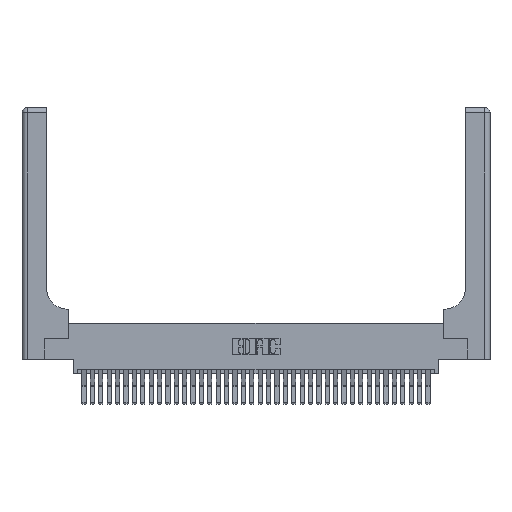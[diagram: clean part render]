
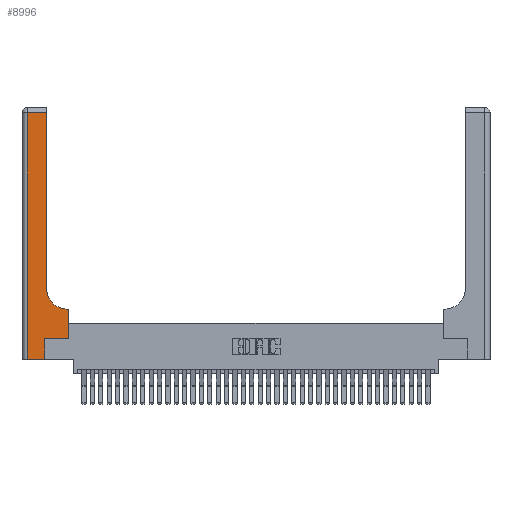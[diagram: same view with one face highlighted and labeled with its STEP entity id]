
A CAD part, top view. The second image highlights one B-rep face of the part: STEP entity #8996.
In plain terms, the highlighted planar face has unit normal (0, 0, 1).
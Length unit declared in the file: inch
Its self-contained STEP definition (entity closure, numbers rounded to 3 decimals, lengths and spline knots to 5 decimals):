
#101 = LINE ( 'NONE', #31288, #15842 ) ;
#147 = LINE ( 'NONE', #14560, #558 ) ;
#292 = DIRECTION ( 'NONE',  ( -1., 0., 0. ) ) ;
#504 = ORIENTED_EDGE ( 'NONE', *, *, #34181, .T. ) ;
#558 = VECTOR ( 'NONE', #29402, 39.37008 ) ;
#624 = PLANE ( 'NONE',  #20999 ) ;
#1263 = DIRECTION ( 'NONE',  ( 1., 0., 0. ) ) ;
#1384 = EDGE_CURVE ( 'NONE', #15365, #7239, #147, .T. ) ;
#1954 = DIRECTION ( 'NONE',  ( 0., 0., -1. ) ) ;
#2042 = ORIENTED_EDGE ( 'NONE', *, *, #28982, .T. ) ;
#2110 = VERTEX_POINT ( 'NONE', #31907 ) ;
#2612 = DIRECTION ( 'NONE',  ( 0., 1., 0. ) ) ;
#3380 = ORIENTED_EDGE ( 'NONE', *, *, #1384, .T. ) ;
#4541 = CARTESIAN_POINT ( 'NONE',  ( 0.5585, 0.6, 0.37 ) ) ;
#6679 = DIRECTION ( 'NONE',  ( -1., 0., 0. ) ) ;
#7239 = VERTEX_POINT ( 'NONE', #7266 ) ;
#7266 = CARTESIAN_POINT ( 'NONE',  ( 0.269, 0., 0.37 ) ) ;
#7744 = CARTESIAN_POINT ( 'NONE',  ( 0., 3., 0.37 ) ) ;
#7892 = CARTESIAN_POINT ( 'NONE',  ( 0.2915, 0.6, 0.37 ) ) ;
#8210 = DIRECTION ( 'NONE',  ( -1., 0., 0. ) ) ;
#8481 = EDGE_CURVE ( 'NONE', #35410, #12416, #36469, .T. ) ;
#8996 = ADVANCED_FACE ( 'NONE', ( #12346 ), #624, .F. ) ;
#9677 = CIRCLE ( 'NONE', #15963, 0.25 ) ;
#10254 = VECTOR ( 'NONE', #22843, 39.37008 ) ;
#10295 = CARTESIAN_POINT ( 'NONE',  ( 0.269, 0.25, 0.37 ) ) ;
#10533 = DIRECTION ( 'NONE',  ( 0., 1., 0. ) ) ;
#11462 = VECTOR ( 'NONE', #10533, 39.37008 ) ;
#12210 = CARTESIAN_POINT ( 'NONE',  ( 0.5415, 0.85, 0.37 ) ) ;
#12346 = FACE_OUTER_BOUND ( 'NONE', #29257, .T. ) ;
#12416 = VERTEX_POINT ( 'NONE', #35075 ) ;
#12736 = VECTOR ( 'NONE', #2612, 39.37008 ) ;
#12944 = ORIENTED_EDGE ( 'NONE', *, *, #18998, .T. ) ;
#13039 = VECTOR ( 'NONE', #21539, 39.37008 ) ;
#14560 = CARTESIAN_POINT ( 'NONE',  ( 0., 0., 0.37 ) ) ;
#15365 = VERTEX_POINT ( 'NONE', #15986 ) ;
#15382 = CARTESIAN_POINT ( 'NONE',  ( 0.269, 0.25, 0.37 ) ) ;
#15471 = ORIENTED_EDGE ( 'NONE', *, *, #28956, .T. ) ;
#15842 = VECTOR ( 'NONE', #16660, 39.37008 ) ;
#15963 = AXIS2_PLACEMENT_3D ( 'NONE', #12210, #32925, #1263 ) ;
#15986 = CARTESIAN_POINT ( 'NONE',  ( 0.06, 0., 0.37 ) ) ;
#16660 = DIRECTION ( 'NONE',  ( 0., -1., 0. ) ) ;
#16808 = LINE ( 'NONE', #7892, #33022 ) ;
#18998 = EDGE_CURVE ( 'NONE', #30718, #38318, #32044, .T. ) ;
#19745 = CARTESIAN_POINT ( 'NONE',  ( 0.269, 0., 0.37 ) ) ;
#20999 = AXIS2_PLACEMENT_3D ( 'NONE', #7744, #1954, #6679 ) ;
#21539 = DIRECTION ( 'NONE',  ( 1., 0., 0. ) ) ;
#22843 = DIRECTION ( 'NONE',  ( 0., 1., 0. ) ) ;
#23670 = VECTOR ( 'NONE', #8210, 39.37008 ) ;
#23707 = LINE ( 'NONE', #19745, #10254 ) ;
#23915 = CARTESIAN_POINT ( 'NONE',  ( 0.2915, 0.85, 0.37 ) ) ;
#24490 = VERTEX_POINT ( 'NONE', #25920 ) ;
#24520 = EDGE_CURVE ( 'NONE', #35234, #24490, #16808, .T. ) ;
#25920 = CARTESIAN_POINT ( 'NONE',  ( 0.5415, 0.6, 0.37 ) ) ;
#26188 = CARTESIAN_POINT ( 'NONE',  ( 0.5585, 0.25, 0.37 ) ) ;
#28956 = EDGE_CURVE ( 'NONE', #7239, #30718, #23707, .T. ) ;
#28982 = EDGE_CURVE ( 'NONE', #2110, #15365, #101, .T. ) ;
#29152 = EDGE_CURVE ( 'NONE', #12416, #2110, #31587, .T. ) ;
#29257 = EDGE_LOOP ( 'NONE', ( #30025, #30339, #2042, #3380, #15471, #12944, #504, #30151, #35249 ) ) ;
#29402 = DIRECTION ( 'NONE',  ( 1., 0., 0. ) ) ;
#30008 = EDGE_CURVE ( 'NONE', #24490, #35410, #9677, .T. ) ;
#30025 = ORIENTED_EDGE ( 'NONE', *, *, #8481, .T. ) ;
#30151 = ORIENTED_EDGE ( 'NONE', *, *, #24520, .T. ) ;
#30339 = ORIENTED_EDGE ( 'NONE', *, *, #29152, .T. ) ;
#30718 = VERTEX_POINT ( 'NONE', #10295 ) ;
#31288 = CARTESIAN_POINT ( 'NONE',  ( 0.06, 3., 0.37 ) ) ;
#31587 = LINE ( 'NONE', #37923, #23670 ) ;
#31907 = CARTESIAN_POINT ( 'NONE',  ( 0.06, 2.94, 0.37 ) ) ;
#32044 = LINE ( 'NONE', #15382, #13039 ) ;
#32925 = DIRECTION ( 'NONE',  ( 0., 0., -1. ) ) ;
#33022 = VECTOR ( 'NONE', #292, 39.37008 ) ;
#33115 = LINE ( 'NONE', #26188, #12736 ) ;
#34181 = EDGE_CURVE ( 'NONE', #38318, #35234, #33115, .T. ) ;
#34693 = CARTESIAN_POINT ( 'NONE',  ( 0.2915, 3., 0.37 ) ) ;
#35075 = CARTESIAN_POINT ( 'NONE',  ( 0.2915, 2.94, 0.37 ) ) ;
#35137 = CARTESIAN_POINT ( 'NONE',  ( 0.5585, 0.25, 0.37 ) ) ;
#35234 = VERTEX_POINT ( 'NONE', #4541 ) ;
#35249 = ORIENTED_EDGE ( 'NONE', *, *, #30008, .T. ) ;
#35410 = VERTEX_POINT ( 'NONE', #23915 ) ;
#36469 = LINE ( 'NONE', #34693, #11462 ) ;
#37923 = CARTESIAN_POINT ( 'NONE',  ( 0., 2.94, 0.37 ) ) ;
#38318 = VERTEX_POINT ( 'NONE', #35137 ) ;
